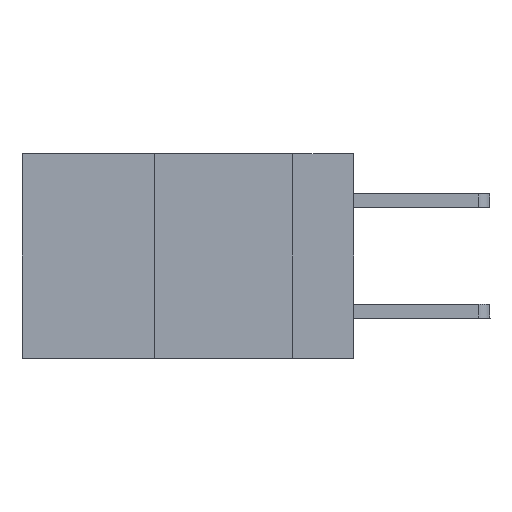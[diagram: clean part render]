
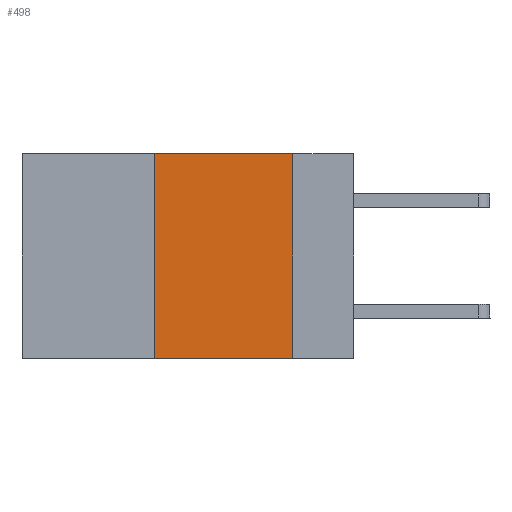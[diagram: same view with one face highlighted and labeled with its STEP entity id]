
A CAD part, left-side view. The second image highlights one B-rep face of the part: STEP entity #498.
In plain terms, the highlighted planar face has unit normal (-1, 0, 0).
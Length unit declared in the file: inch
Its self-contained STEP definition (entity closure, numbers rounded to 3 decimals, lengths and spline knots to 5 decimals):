
#31 = VECTOR ( 'NONE', #898, 39.37008 ) ;
#498 = ADVANCED_FACE ( 'NONE', ( #6243 ), #10796, .F. ) ;
#824 = CARTESIAN_POINT ( 'NONE',  ( 0., 0.36, 0. ) ) ;
#898 = DIRECTION ( 'NONE',  ( 0., 0., -1. ) ) ;
#1122 = ORIENTED_EDGE ( 'NONE', *, *, #13868, .F. ) ;
#1449 = CARTESIAN_POINT ( 'NONE',  ( 0., 0.6, -0.37 ) ) ;
#2165 = CARTESIAN_POINT ( 'NONE',  ( 0., 0.11, 0. ) ) ;
#2437 = VECTOR ( 'NONE', #10508, 39.37008 ) ;
#3907 = CARTESIAN_POINT ( 'NONE',  ( 0., 0.6, 0. ) ) ;
#5807 = CARTESIAN_POINT ( 'NONE',  ( 0., 0.36, 0. ) ) ;
#5952 = LINE ( 'NONE', #5807, #2437 ) ;
#6208 = DIRECTION ( 'NONE',  ( 0., -1., 0. ) ) ;
#6243 = FACE_OUTER_BOUND ( 'NONE', #6839, .T. ) ;
#6276 = LINE ( 'NONE', #3907, #13407 ) ;
#6412 = CARTESIAN_POINT ( 'NONE',  ( 0., 0.11, 0. ) ) ;
#6619 = VERTEX_POINT ( 'NONE', #2165 ) ;
#6639 = CARTESIAN_POINT ( 'NONE',  ( 0., 0.36, -0.37 ) ) ;
#6839 = EDGE_LOOP ( 'NONE', ( #7747, #9080, #1122, #7298 ) ) ;
#7298 = ORIENTED_EDGE ( 'NONE', *, *, #13452, .T. ) ;
#7747 = ORIENTED_EDGE ( 'NONE', *, *, #11050, .F. ) ;
#7796 = EDGE_CURVE ( 'NONE', #11091, #6619, #6276, .T. ) ;
#8821 = CARTESIAN_POINT ( 'NONE',  ( 0., 0.11, -0.37 ) ) ;
#9080 = ORIENTED_EDGE ( 'NONE', *, *, #7796, .F. ) ;
#9531 = CARTESIAN_POINT ( 'NONE',  ( 0., 0.6, 0. ) ) ;
#9682 = DIRECTION ( 'NONE',  ( 1., 0., 0. ) ) ;
#9970 = AXIS2_PLACEMENT_3D ( 'NONE', #9531, #9682, #14061 ) ;
#10051 = VECTOR ( 'NONE', #6208, 39.37008 ) ;
#10508 = DIRECTION ( 'NONE',  ( 0., 0., 1. ) ) ;
#10796 = PLANE ( 'NONE',  #9970 ) ;
#11041 = LINE ( 'NONE', #6412, #31 ) ;
#11050 = EDGE_CURVE ( 'NONE', #6619, #11906, #11041, .T. ) ;
#11091 = VERTEX_POINT ( 'NONE', #824 ) ;
#11906 = VERTEX_POINT ( 'NONE', #8821 ) ;
#12463 = VERTEX_POINT ( 'NONE', #6639 ) ;
#13407 = VECTOR ( 'NONE', #14171, 39.37008 ) ;
#13452 = EDGE_CURVE ( 'NONE', #12463, #11906, #13890, .T. ) ;
#13868 = EDGE_CURVE ( 'NONE', #12463, #11091, #5952, .T. ) ;
#13890 = LINE ( 'NONE', #1449, #10051 ) ;
#14061 = DIRECTION ( 'NONE',  ( 0., 0., -1. ) ) ;
#14171 = DIRECTION ( 'NONE',  ( 0., -1., 0. ) ) ;
